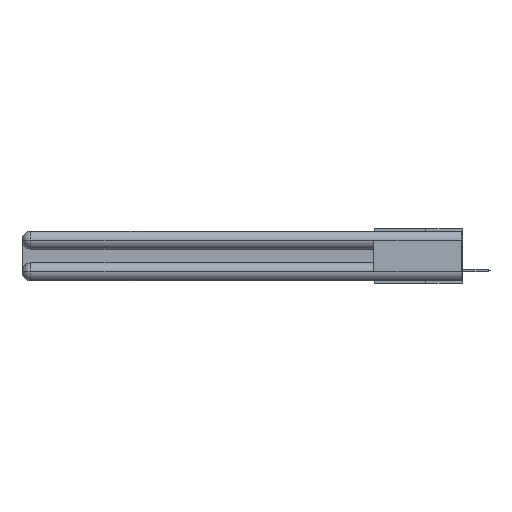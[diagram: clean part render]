
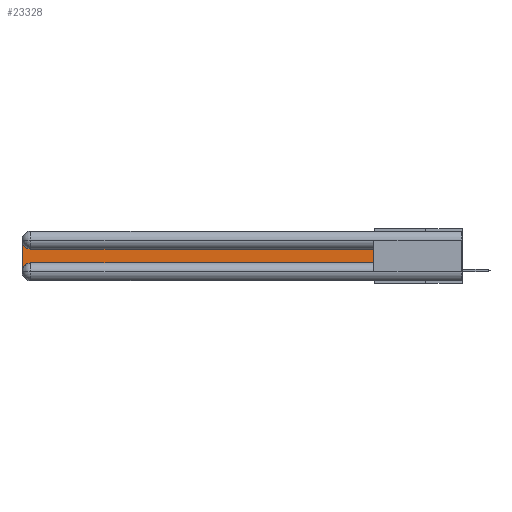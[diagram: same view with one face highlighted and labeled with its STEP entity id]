
A CAD part, left-side view. The second image highlights one B-rep face of the part: STEP entity #23328.
In plain terms, the highlighted planar face has unit normal (-1, 0, 0).
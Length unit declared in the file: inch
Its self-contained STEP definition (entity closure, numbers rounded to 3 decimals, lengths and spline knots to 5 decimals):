
#1056 = ORIENTED_EDGE ( 'NONE', *, *, #22222, .T. ) ;
#1101 = DIRECTION ( 'NONE',  ( 0., 1., 0. ) ) ;
#2129 = LINE ( 'NONE', #27236, #25068 ) ;
#2572 = DIRECTION ( 'NONE',  ( 1., 0., 0. ) ) ;
#2832 = VERTEX_POINT ( 'NONE', #25111 ) ;
#3811 = VERTEX_POINT ( 'NONE', #26192 ) ;
#4408 = AXIS2_PLACEMENT_3D ( 'NONE', #9367, #2572, #25396 ) ;
#4624 = VERTEX_POINT ( 'NONE', #18298 ) ;
#5001 = EDGE_CURVE ( 'NONE', #3811, #8883, #8037, .T. ) ;
#6416 = DIRECTION ( 'NONE',  ( 1., 0., 0. ) ) ;
#7010 = VECTOR ( 'NONE', #1101, 39.37008 ) ;
#7044 = PLANE ( 'NONE',  #4408 ) ;
#7121 = VERTEX_POINT ( 'NONE', #10484 ) ;
#7267 = ORIENTED_EDGE ( 'NONE', *, *, #28656, .T. ) ;
#8037 = CIRCLE ( 'NONE', #14091, 0.06 ) ;
#8456 = VECTOR ( 'NONE', #18601, 39.37008 ) ;
#8883 = VERTEX_POINT ( 'NONE', #17710 ) ;
#9000 = DIRECTION ( 'NONE',  ( 0., -1., 0. ) ) ;
#9367 = CARTESIAN_POINT ( 'NONE',  ( 0.075, 3., -0.1225 ) ) ;
#10484 = CARTESIAN_POINT ( 'NONE',  ( 0.075, 0.6, -0.1225 ) ) ;
#10551 = ORIENTED_EDGE ( 'NONE', *, *, #16330, .T. ) ;
#11459 = VECTOR ( 'NONE', #15151, 39.37008 ) ;
#12190 = LINE ( 'NONE', #14861, #11459 ) ;
#12374 = ORIENTED_EDGE ( 'NONE', *, *, #16045, .T. ) ;
#12543 = EDGE_CURVE ( 'NONE', #4624, #7121, #13511, .T. ) ;
#12743 = CARTESIAN_POINT ( 'NONE',  ( 0.075, 0.6, -0.1225 ) ) ;
#12773 = DIRECTION ( 'NONE',  ( 1., 0., 0. ) ) ;
#13511 = LINE ( 'NONE', #20607, #8456 ) ;
#13518 = ORIENTED_EDGE ( 'NONE', *, *, #12543, .T. ) ;
#14091 = AXIS2_PLACEMENT_3D ( 'NONE', #15093, #12773, #17459 ) ;
#14861 = CARTESIAN_POINT ( 'NONE',  ( 0.075, 3., -0.2175 ) ) ;
#15093 = CARTESIAN_POINT ( 'NONE',  ( 0.075, 2.94, -0.2775 ) ) ;
#15151 = DIRECTION ( 'NONE',  ( 0., 0., -1. ) ) ;
#16045 = EDGE_CURVE ( 'NONE', #26195, #3811, #12190, .T. ) ;
#16330 = EDGE_CURVE ( 'NONE', #8883, #4624, #2129, .T. ) ;
#16704 = LINE ( 'NONE', #12743, #7010 ) ;
#16745 = CIRCLE ( 'NONE', #22007, 0.06 ) ;
#17459 = DIRECTION ( 'NONE',  ( 0., 0., -1. ) ) ;
#17710 = CARTESIAN_POINT ( 'NONE',  ( 0.075, 2.94, -0.2175 ) ) ;
#18298 = CARTESIAN_POINT ( 'NONE',  ( 0.075, 0.6, -0.2175 ) ) ;
#18601 = DIRECTION ( 'NONE',  ( 0., 0., 1. ) ) ;
#20129 = CARTESIAN_POINT ( 'NONE',  ( 0.075, 2.94, -0.0625 ) ) ;
#20607 = CARTESIAN_POINT ( 'NONE',  ( 0.075, 0.6, -0.2175 ) ) ;
#21143 = EDGE_LOOP ( 'NONE', ( #7267, #1056, #12374, #25592, #10551, #13518 ) ) ;
#22007 = AXIS2_PLACEMENT_3D ( 'NONE', #20129, #6416, #24765 ) ;
#22222 = EDGE_CURVE ( 'NONE', #2832, #26195, #16745, .T. ) ;
#23328 = ADVANCED_FACE ( 'NONE', ( #24905 ), #7044, .F. ) ;
#24765 = DIRECTION ( 'NONE',  ( 0., 0., -1. ) ) ;
#24905 = FACE_OUTER_BOUND ( 'NONE', #21143, .T. ) ;
#25068 = VECTOR ( 'NONE', #9000, 39.37008 ) ;
#25111 = CARTESIAN_POINT ( 'NONE',  ( 0.075, 2.94, -0.1225 ) ) ;
#25396 = DIRECTION ( 'NONE',  ( 0., 0., -1. ) ) ;
#25592 = ORIENTED_EDGE ( 'NONE', *, *, #5001, .T. ) ;
#26192 = CARTESIAN_POINT ( 'NONE',  ( 0.075, 3., -0.2775 ) ) ;
#26195 = VERTEX_POINT ( 'NONE', #28488 ) ;
#27236 = CARTESIAN_POINT ( 'NONE',  ( 0.075, 0.6, -0.2175 ) ) ;
#28488 = CARTESIAN_POINT ( 'NONE',  ( 0.075, 3., -0.0625 ) ) ;
#28656 = EDGE_CURVE ( 'NONE', #7121, #2832, #16704, .T. ) ;
